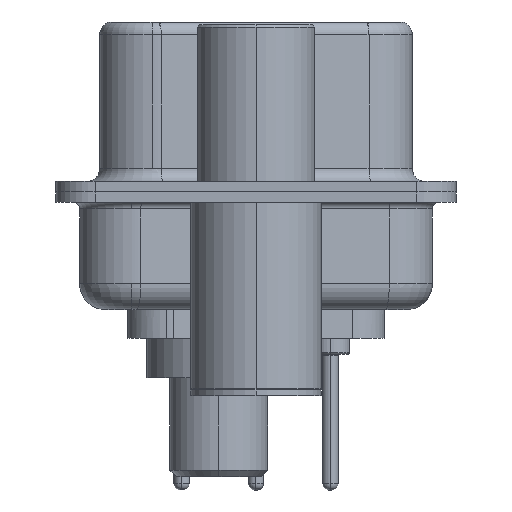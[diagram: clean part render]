
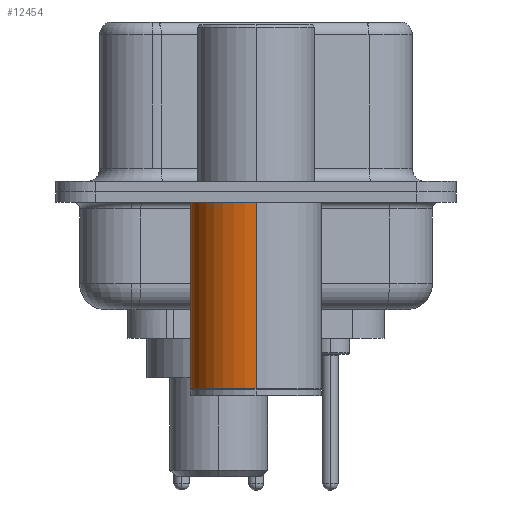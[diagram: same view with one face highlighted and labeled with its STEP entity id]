
A CAD part, left-side view. The second image highlights one B-rep face of the part: STEP entity #12454.
In plain terms, the highlighted cylindrical face has radius 2.5 mm (diameter 5 mm), a partial arc.
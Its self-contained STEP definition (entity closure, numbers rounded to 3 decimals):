
#329 = DIRECTION ( 'NONE',  ( 0., 0., 1. ) ) ;
#1347 = CARTESIAN_POINT ( 'NONE',  ( 0., 0., 0.581 ) ) ;
#3069 = EDGE_LOOP ( 'NONE', ( #13770, #13164, #9855, #3486 ) ) ;
#3486 = ORIENTED_EDGE ( 'NONE', *, *, #22623, .F. ) ;
#3554 = CARTESIAN_POINT ( 'NONE',  ( -2.5, 0., 0.581 ) ) ;
#5641 = DIRECTION ( 'NONE',  ( 1., 0., 0. ) ) ;
#5895 = CARTESIAN_POINT ( 'NONE',  ( -2.5, 0., -7.525 ) ) ;
#8321 = LINE ( 'NONE', #27009, #24400 ) ;
#9499 = DIRECTION ( 'NONE',  ( 0., 0., 1. ) ) ;
#9855 = ORIENTED_EDGE ( 'NONE', *, *, #24807, .F. ) ;
#9958 = VERTEX_POINT ( 'NONE', #16585 ) ;
#10525 = CIRCLE ( 'NONE', #25546, 2.5 ) ;
#11606 = CARTESIAN_POINT ( 'NONE',  ( -2.5, 0., -0.4 ) ) ;
#12454 = ADVANCED_FACE ( 'NONE', ( #27607 ), #15982, .T. ) ;
#13164 = ORIENTED_EDGE ( 'NONE', *, *, #14888, .T. ) ;
#13357 = CARTESIAN_POINT ( 'NONE',  ( 0., 0., -7.525 ) ) ;
#13737 = EDGE_CURVE ( 'NONE', #24569, #25638, #10525, .T. ) ;
#13770 = ORIENTED_EDGE ( 'NONE', *, *, #13737, .T. ) ;
#14888 = EDGE_CURVE ( 'NONE', #25638, #16400, #25823, .T. ) ;
#15511 = DIRECTION ( 'NONE',  ( 1., 0., 0. ) ) ;
#15982 = CYLINDRICAL_SURFACE ( 'NONE', #17984, 2.5 ) ;
#15997 = CARTESIAN_POINT ( 'NONE',  ( 2.5, 0., -7.525 ) ) ;
#16162 = AXIS2_PLACEMENT_3D ( 'NONE', #22576, #9499, #24804 ) ;
#16400 = VERTEX_POINT ( 'NONE', #11606 ) ;
#16475 = DIRECTION ( 'NONE',  ( 0., 0., 1. ) ) ;
#16585 = CARTESIAN_POINT ( 'NONE',  ( 2.5, 0., -0.4 ) ) ;
#17059 = CIRCLE ( 'NONE', #16162, 2.5 ) ;
#17984 = AXIS2_PLACEMENT_3D ( 'NONE', #1347, #20885, #5641 ) ;
#20885 = DIRECTION ( 'NONE',  ( 0., 0., 1. ) ) ;
#22576 = CARTESIAN_POINT ( 'NONE',  ( 0., 0., -0.4 ) ) ;
#22623 = EDGE_CURVE ( 'NONE', #24569, #9958, #8321, .T. ) ;
#24400 = VECTOR ( 'NONE', #24844, 1000. ) ;
#24569 = VERTEX_POINT ( 'NONE', #15997 ) ;
#24804 = DIRECTION ( 'NONE',  ( 1., 0., 0. ) ) ;
#24807 = EDGE_CURVE ( 'NONE', #9958, #16400, #17059, .T. ) ;
#24844 = DIRECTION ( 'NONE',  ( 0., 0., 1. ) ) ;
#25149 = VECTOR ( 'NONE', #16475, 1000. ) ;
#25546 = AXIS2_PLACEMENT_3D ( 'NONE', #13357, #329, #15511 ) ;
#25638 = VERTEX_POINT ( 'NONE', #5895 ) ;
#25823 = LINE ( 'NONE', #3554, #25149 ) ;
#27009 = CARTESIAN_POINT ( 'NONE',  ( 2.5, 0., 0.581 ) ) ;
#27607 = FACE_OUTER_BOUND ( 'NONE', #3069, .T. ) ;
